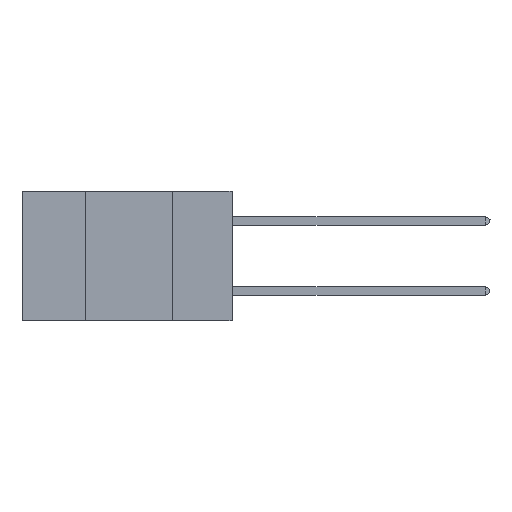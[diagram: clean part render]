
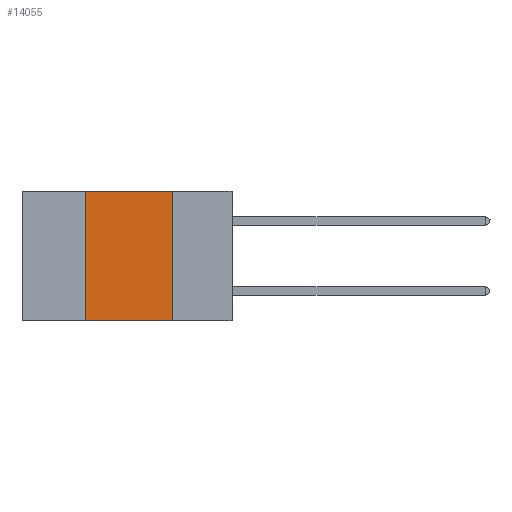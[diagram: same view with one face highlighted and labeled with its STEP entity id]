
A CAD part, left-side view. The second image highlights one B-rep face of the part: STEP entity #14055.
In plain terms, the highlighted planar face has unit normal (-1, 0, 0).
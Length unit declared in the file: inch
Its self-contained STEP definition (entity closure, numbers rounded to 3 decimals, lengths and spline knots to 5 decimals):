
#2533 = CARTESIAN_POINT ( 'NONE',  ( 0., 0.42, -0.37 ) ) ;
#3325 = PLANE ( 'NONE',  #8271 ) ;
#8271 = AXIS2_PLACEMENT_3D ( 'NONE', #23520, #37284, #44136 ) ;
#9322 = ORIENTED_EDGE ( 'NONE', *, *, #31804, .T. ) ;
#11340 = VECTOR ( 'NONE', #34118, 39.37008 ) ;
#12955 = CARTESIAN_POINT ( 'NONE',  ( 0., 0.6, 0. ) ) ;
#14055 = ADVANCED_FACE ( 'NONE', ( #33850 ), #3325, .F. ) ;
#14768 = CARTESIAN_POINT ( 'NONE',  ( 0., 0.6, -0.37 ) ) ;
#17712 = ORIENTED_EDGE ( 'NONE', *, *, #30977, .F. ) ;
#18235 = CARTESIAN_POINT ( 'NONE',  ( 0., 0.17, -0.37 ) ) ;
#19351 = LINE ( 'NONE', #14768, #35425 ) ;
#20916 = VERTEX_POINT ( 'NONE', #18235 ) ;
#23064 = CARTESIAN_POINT ( 'NONE',  ( 0., 0.17, 0. ) ) ;
#23520 = CARTESIAN_POINT ( 'NONE',  ( 0., 0.6, 0. ) ) ;
#23569 = CARTESIAN_POINT ( 'NONE',  ( 0., 0.17, 0. ) ) ;
#25900 = EDGE_CURVE ( 'NONE', #29754, #40322, #30373, .T. ) ;
#26945 = DIRECTION ( 'NONE',  ( 0., -1., 0. ) ) ;
#27953 = LINE ( 'NONE', #45131, #28349 ) ;
#28349 = VECTOR ( 'NONE', #34603, 39.37008 ) ;
#28719 = EDGE_LOOP ( 'NONE', ( #17712, #37408, #41648, #9322 ) ) ;
#29754 = VERTEX_POINT ( 'NONE', #44173 ) ;
#30373 = LINE ( 'NONE', #12955, #42156 ) ;
#30977 = EDGE_CURVE ( 'NONE', #40322, #20916, #44855, .T. ) ;
#31804 = EDGE_CURVE ( 'NONE', #42636, #20916, #19351, .T. ) ;
#33850 = FACE_OUTER_BOUND ( 'NONE', #28719, .T. ) ;
#34118 = DIRECTION ( 'NONE',  ( 0., 0., -1. ) ) ;
#34603 = DIRECTION ( 'NONE',  ( 0., 0., 1. ) ) ;
#35425 = VECTOR ( 'NONE', #36557, 39.37008 ) ;
#35639 = EDGE_CURVE ( 'NONE', #42636, #29754, #27953, .T. ) ;
#36557 = DIRECTION ( 'NONE',  ( 0., -1., 0. ) ) ;
#37284 = DIRECTION ( 'NONE',  ( 1., 0., 0. ) ) ;
#37408 = ORIENTED_EDGE ( 'NONE', *, *, #25900, .F. ) ;
#40322 = VERTEX_POINT ( 'NONE', #23064 ) ;
#41648 = ORIENTED_EDGE ( 'NONE', *, *, #35639, .F. ) ;
#42156 = VECTOR ( 'NONE', #26945, 39.37008 ) ;
#42636 = VERTEX_POINT ( 'NONE', #2533 ) ;
#44136 = DIRECTION ( 'NONE',  ( 0., 0., -1. ) ) ;
#44173 = CARTESIAN_POINT ( 'NONE',  ( 0., 0.42, 0. ) ) ;
#44855 = LINE ( 'NONE', #23569, #11340 ) ;
#45131 = CARTESIAN_POINT ( 'NONE',  ( 0., 0.42, 0. ) ) ;
